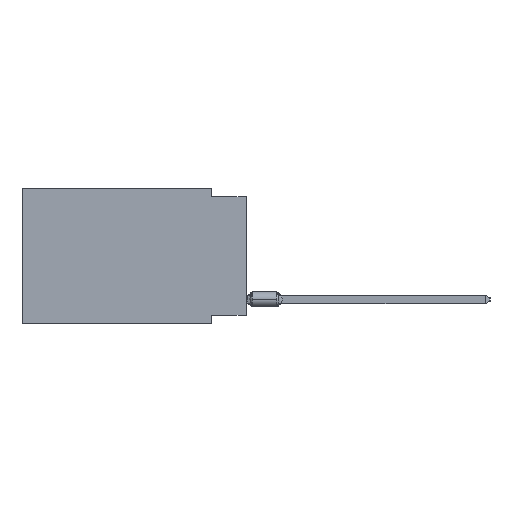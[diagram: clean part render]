
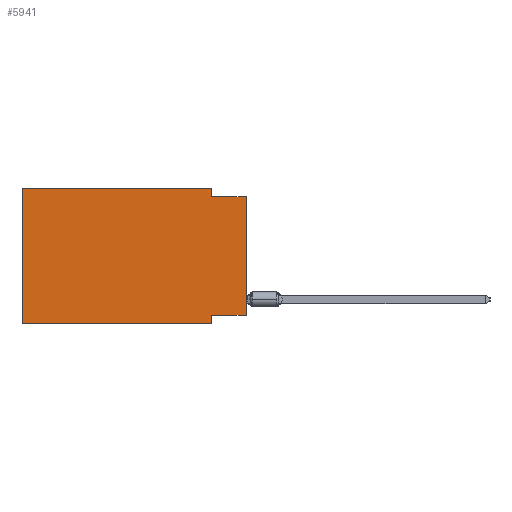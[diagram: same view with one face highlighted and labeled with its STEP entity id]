
A CAD part, left-side view. The second image highlights one B-rep face of the part: STEP entity #5941.
In plain terms, the highlighted planar face has unit normal (-1, 0, 0).
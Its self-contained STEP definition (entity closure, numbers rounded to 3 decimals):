
#1264 = VECTOR ( 'NONE', #17672, 1000. ) ;
#1462 = CARTESIAN_POINT ( 'NONE',  ( 0., 16.383, 0. ) ) ;
#2215 = DIRECTION ( 'NONE',  ( 1., 0., 0. ) ) ;
#2478 = CARTESIAN_POINT ( 'NONE',  ( 0., 0., -0.635 ) ) ;
#2931 = EDGE_CURVE ( 'NONE', #15210, #27617, #33634, .T. ) ;
#3456 = VECTOR ( 'NONE', #15304, 1000. ) ;
#3831 = VERTEX_POINT ( 'NONE', #39926 ) ;
#4836 = CARTESIAN_POINT ( 'NONE',  ( 0., 2.54, -9.906 ) ) ;
#5199 = VERTEX_POINT ( 'NONE', #6751 ) ;
#5216 = DIRECTION ( 'NONE',  ( 0., -1., 0. ) ) ;
#5366 = FACE_OUTER_BOUND ( 'NONE', #7854, .T. ) ;
#5941 = ADVANCED_FACE ( 'NONE', ( #5366 ), #25362, .F. ) ;
#6751 = CARTESIAN_POINT ( 'NONE',  ( 0., 2.54, -0.635 ) ) ;
#7064 = EDGE_CURVE ( 'NONE', #41151, #5199, #20975, .T. ) ;
#7453 = AXIS2_PLACEMENT_3D ( 'NONE', #41073, #2215, #41289 ) ;
#7854 = EDGE_LOOP ( 'NONE', ( #9677, #31212, #14432, #13298, #22111, #11670, #41087, #21806 ) ) ;
#8748 = EDGE_CURVE ( 'NONE', #20989, #27617, #34471, .T. ) ;
#9016 = CARTESIAN_POINT ( 'NONE',  ( 0., 16.383, 0. ) ) ;
#9596 = CARTESIAN_POINT ( 'NONE',  ( 0., 16.383, -9.906 ) ) ;
#9677 = ORIENTED_EDGE ( 'NONE', *, *, #35823, .T. ) ;
#11627 = VECTOR ( 'NONE', #12405, 1000. ) ;
#11670 = ORIENTED_EDGE ( 'NONE', *, *, #8748, .T. ) ;
#12014 = VERTEX_POINT ( 'NONE', #20970 ) ;
#12405 = DIRECTION ( 'NONE',  ( 0., -1., 0. ) ) ;
#13032 = DIRECTION ( 'NONE',  ( 0., 1., 0. ) ) ;
#13298 = ORIENTED_EDGE ( 'NONE', *, *, #29116, .F. ) ;
#14380 = EDGE_CURVE ( 'NONE', #20989, #3831, #26911, .T. ) ;
#14432 = ORIENTED_EDGE ( 'NONE', *, *, #7064, .F. ) ;
#15210 = VERTEX_POINT ( 'NONE', #41457 ) ;
#15304 = DIRECTION ( 'NONE',  ( 0., -1., 0. ) ) ;
#16675 = CARTESIAN_POINT ( 'NONE',  ( 0., 0., 0. ) ) ;
#17145 = VECTOR ( 'NONE', #5216, 1000. ) ;
#17190 = DIRECTION ( 'NONE',  ( 0., 0., -1. ) ) ;
#17672 = DIRECTION ( 'NONE',  ( 0., 0., -1. ) ) ;
#17940 = EDGE_CURVE ( 'NONE', #5199, #39498, #40919, .T. ) ;
#18259 = LINE ( 'NONE', #9016, #17145 ) ;
#18291 = CARTESIAN_POINT ( 'NONE',  ( 0., 16.383, -9.906 ) ) ;
#19561 = CARTESIAN_POINT ( 'NONE',  ( 0., 0., -9.271 ) ) ;
#20970 = CARTESIAN_POINT ( 'NONE',  ( 0., 0., -9.271 ) ) ;
#20975 = LINE ( 'NONE', #40073, #25041 ) ;
#20989 = VERTEX_POINT ( 'NONE', #9596 ) ;
#21806 = ORIENTED_EDGE ( 'NONE', *, *, #23055, .F. ) ;
#22111 = ORIENTED_EDGE ( 'NONE', *, *, #14380, .F. ) ;
#23055 = EDGE_CURVE ( 'NONE', #12014, #15210, #38653, .T. ) ;
#25041 = VECTOR ( 'NONE', #17190, 1000. ) ;
#25362 = PLANE ( 'NONE',  #7453 ) ;
#26911 = LINE ( 'NONE', #1462, #39935 ) ;
#26999 = CARTESIAN_POINT ( 'NONE',  ( 0., 2.54, -9.906 ) ) ;
#27617 = VERTEX_POINT ( 'NONE', #26999 ) ;
#29116 = EDGE_CURVE ( 'NONE', #3831, #41151, #18259, .T. ) ;
#31212 = ORIENTED_EDGE ( 'NONE', *, *, #17940, .F. ) ;
#32844 = LINE ( 'NONE', #16675, #40917 ) ;
#33634 = LINE ( 'NONE', #4836, #1264 ) ;
#34471 = LINE ( 'NONE', #18291, #11627 ) ;
#35134 = CARTESIAN_POINT ( 'NONE',  ( 0., 0., -0.635 ) ) ;
#35779 = DIRECTION ( 'NONE',  ( 0., 0., 1. ) ) ;
#35823 = EDGE_CURVE ( 'NONE', #12014, #39498, #32844, .T. ) ;
#37378 = VECTOR ( 'NONE', #13032, 1000. ) ;
#37828 = CARTESIAN_POINT ( 'NONE',  ( 0., 2.54, 0. ) ) ;
#38653 = LINE ( 'NONE', #19561, #37378 ) ;
#39498 = VERTEX_POINT ( 'NONE', #35134 ) ;
#39696 = DIRECTION ( 'NONE',  ( 0., 0., 1. ) ) ;
#39926 = CARTESIAN_POINT ( 'NONE',  ( 0., 16.383, 0. ) ) ;
#39935 = VECTOR ( 'NONE', #39696, 1000. ) ;
#40073 = CARTESIAN_POINT ( 'NONE',  ( 0., 2.54, 0. ) ) ;
#40917 = VECTOR ( 'NONE', #35779, 1000. ) ;
#40919 = LINE ( 'NONE', #2478, #3456 ) ;
#41073 = CARTESIAN_POINT ( 'NONE',  ( 0., 16.383, 0. ) ) ;
#41087 = ORIENTED_EDGE ( 'NONE', *, *, #2931, .F. ) ;
#41151 = VERTEX_POINT ( 'NONE', #37828 ) ;
#41289 = DIRECTION ( 'NONE',  ( 0., 0., -1. ) ) ;
#41457 = CARTESIAN_POINT ( 'NONE',  ( 0., 2.54, -9.271 ) ) ;
